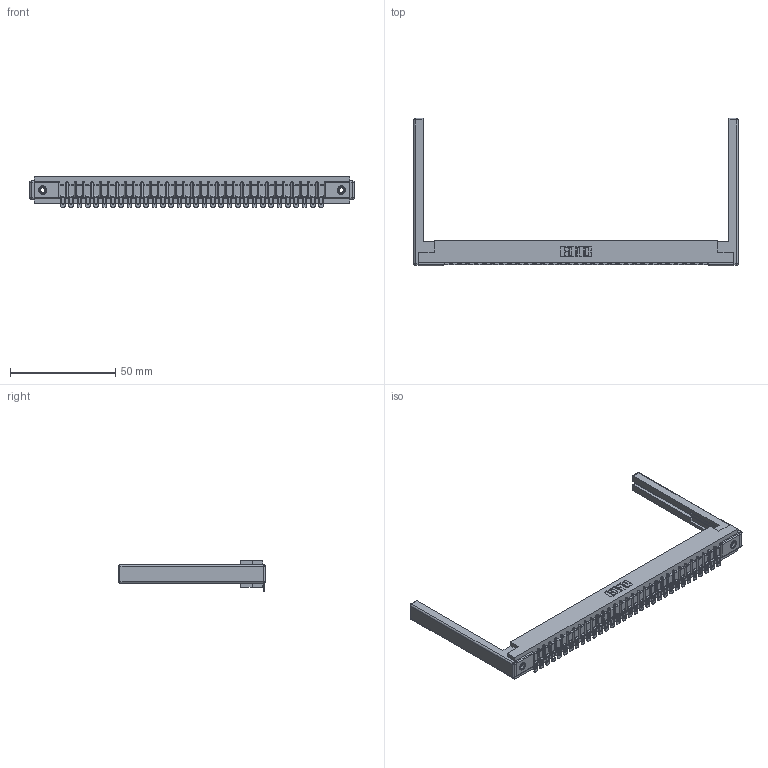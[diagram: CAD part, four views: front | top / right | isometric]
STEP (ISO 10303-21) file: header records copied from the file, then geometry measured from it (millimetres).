
FILE_DESCRIPTION (( 'STEP AP203' ), '1' );
FILE_NAME ('307-032-454-168.STEP', '2020-09-28T17:04:50', ( '' ), ( '' ), 'SwSTEP 2.0', 'SolidWorks 2020', '' );
FILE_SCHEMA (( 'CONFIG_CONTROL_DESIGN' ));
Length unit declared in the file: inch
Products named in the file (5): 307-032-454-168; 307-290-002_554; 345-250-001_345-250-001-102; 307-220-068; 307 Part_.156 Dia Mounting Holes
Assembly tree (37 placements, depth 2):
  307-032-454-168
    307 Part_.156 Dia Mounting Holes
    307-290-002_554  x32
    307-220-068  x2
    345-250-001_345-250-001-102  x2
Bounding box: 154.23 x 69.98 x 14.52 mm (x, y, z)
Volume: 20819 mm3; surface area: 24538.2 mm2
Topology: 37 solids, 37 shells, 2897 faces, 8809 edges, 5762 vertices
Faces by surface type: plane 1630, cylinder 1177, sphere 74, cone 12, torus 4
Entity records: 32390 total; most frequent: CARTESIAN_POINT 5427, ORIENTED_EDGE 5406, DIRECTION 5301, EDGE_CURVE 2703, LINE 2057, VECTOR 2057, VERTEX_POINT 1748, AXIS2_PLACEMENT_3D 1622
